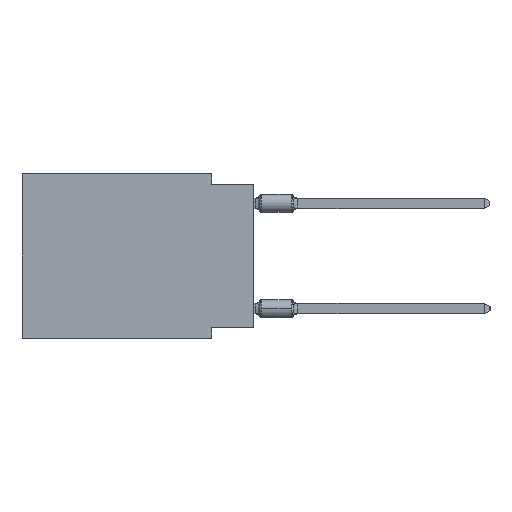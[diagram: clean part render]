
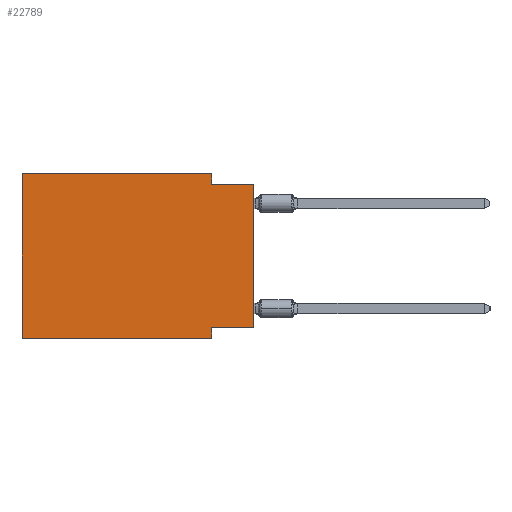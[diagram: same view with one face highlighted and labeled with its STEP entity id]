
A CAD part, left-side view. The second image highlights one B-rep face of the part: STEP entity #22789.
In plain terms, the highlighted planar face has unit normal (-1, 0, 0).
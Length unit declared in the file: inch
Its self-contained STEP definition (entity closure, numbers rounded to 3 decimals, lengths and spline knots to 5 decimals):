
#131 = CARTESIAN_POINT ( 'NONE',  ( 0., 0.1, -0.39 ) ) ;
#593 = LINE ( 'NONE', #9937, #12192 ) ;
#1393 = CARTESIAN_POINT ( 'NONE',  ( 0., 0.1, 0. ) ) ;
#1691 = ORIENTED_EDGE ( 'NONE', *, *, #12600, .F. ) ;
#2046 = ORIENTED_EDGE ( 'NONE', *, *, #15330, .F. ) ;
#2110 = DIRECTION ( 'NONE',  ( 0., 0., -1. ) ) ;
#2387 = VERTEX_POINT ( 'NONE', #2949 ) ;
#2538 = ORIENTED_EDGE ( 'NONE', *, *, #18547, .F. ) ;
#2949 = CARTESIAN_POINT ( 'NONE',  ( 0., 0.55, -0.39 ) ) ;
#3519 = VERTEX_POINT ( 'NONE', #9788 ) ;
#3771 = ORIENTED_EDGE ( 'NONE', *, *, #26966, .F. ) ;
#4099 = LINE ( 'NONE', #29388, #11562 ) ;
#5798 = ORIENTED_EDGE ( 'NONE', *, *, #21967, .T. ) ;
#5980 = ORIENTED_EDGE ( 'NONE', *, *, #15368, .T. ) ;
#7129 = VERTEX_POINT ( 'NONE', #11928 ) ;
#7534 = CARTESIAN_POINT ( 'NONE',  ( 0., 0., -0.365 ) ) ;
#7773 = VECTOR ( 'NONE', #2110, 39.37008 ) ;
#7904 = DIRECTION ( 'NONE',  ( 0., -1., 0. ) ) ;
#8086 = VERTEX_POINT ( 'NONE', #22622 ) ;
#9294 = CARTESIAN_POINT ( 'NONE',  ( 0., 0.1, 0. ) ) ;
#9782 = CARTESIAN_POINT ( 'NONE',  ( 0., 0.55, -0.39 ) ) ;
#9788 = CARTESIAN_POINT ( 'NONE',  ( 0., 0.55, 0. ) ) ;
#9811 = DIRECTION ( 'NONE',  ( 0., 0., 1. ) ) ;
#9903 = EDGE_CURVE ( 'NONE', #2387, #3519, #4099, .T. ) ;
#9937 = CARTESIAN_POINT ( 'NONE',  ( 0., 0., -0.365 ) ) ;
#10056 = VERTEX_POINT ( 'NONE', #27062 ) ;
#10591 = DIRECTION ( 'NONE',  ( 0., 0., -1. ) ) ;
#11188 = DIRECTION ( 'NONE',  ( 0., 0., 1. ) ) ;
#11562 = VECTOR ( 'NONE', #11188, 39.37008 ) ;
#11720 = DIRECTION ( 'NONE',  ( 0., -1., 0. ) ) ;
#11928 = CARTESIAN_POINT ( 'NONE',  ( 0., 0.1, -0.025 ) ) ;
#12192 = VECTOR ( 'NONE', #28292, 39.37008 ) ;
#12600 = EDGE_CURVE ( 'NONE', #20473, #13863, #593, .T. ) ;
#13360 = EDGE_LOOP ( 'NONE', ( #5798, #2538, #3771, #13796, #21833, #5980, #2046, #1691 ) ) ;
#13619 = DIRECTION ( 'NONE',  ( 1., 0., 0. ) ) ;
#13796 = ORIENTED_EDGE ( 'NONE', *, *, #23709, .F. ) ;
#13863 = VERTEX_POINT ( 'NONE', #27448 ) ;
#14271 = VECTOR ( 'NONE', #11720, 39.37008 ) ;
#14648 = LINE ( 'NONE', #16907, #27155 ) ;
#15330 = EDGE_CURVE ( 'NONE', #13863, #10056, #22752, .T. ) ;
#15368 = EDGE_CURVE ( 'NONE', #2387, #10056, #23639, .T. ) ;
#15563 = FACE_OUTER_BOUND ( 'NONE', #13360, .T. ) ;
#16907 = CARTESIAN_POINT ( 'NONE',  ( 0., 0., 0. ) ) ;
#18547 = EDGE_CURVE ( 'NONE', #7129, #8086, #28783, .T. ) ;
#18630 = LINE ( 'NONE', #22714, #14271 ) ;
#19469 = CARTESIAN_POINT ( 'NONE',  ( 0., 0., -0.025 ) ) ;
#19980 = AXIS2_PLACEMENT_3D ( 'NONE', #24577, #13619, #20506 ) ;
#20473 = VERTEX_POINT ( 'NONE', #7534 ) ;
#20506 = DIRECTION ( 'NONE',  ( 0., 0., -1. ) ) ;
#20609 = VECTOR ( 'NONE', #10591, 39.37008 ) ;
#21382 = DIRECTION ( 'NONE',  ( 0., -1., 0. ) ) ;
#21747 = LINE ( 'NONE', #1393, #20609 ) ;
#21833 = ORIENTED_EDGE ( 'NONE', *, *, #9903, .F. ) ;
#21967 = EDGE_CURVE ( 'NONE', #20473, #8086, #14648, .T. ) ;
#22202 = PLANE ( 'NONE',  #19980 ) ;
#22622 = CARTESIAN_POINT ( 'NONE',  ( 0., 0., -0.025 ) ) ;
#22714 = CARTESIAN_POINT ( 'NONE',  ( 0., 0.55, 0. ) ) ;
#22752 = LINE ( 'NONE', #131, #7773 ) ;
#22789 = ADVANCED_FACE ( 'NONE', ( #15563 ), #22202, .F. ) ;
#23639 = LINE ( 'NONE', #9782, #27449 ) ;
#23709 = EDGE_CURVE ( 'NONE', #3519, #23807, #18630, .T. ) ;
#23807 = VERTEX_POINT ( 'NONE', #9294 ) ;
#24577 = CARTESIAN_POINT ( 'NONE',  ( 0., 0.55, 0. ) ) ;
#26966 = EDGE_CURVE ( 'NONE', #23807, #7129, #21747, .T. ) ;
#27062 = CARTESIAN_POINT ( 'NONE',  ( 0., 0.1, -0.39 ) ) ;
#27155 = VECTOR ( 'NONE', #9811, 39.37008 ) ;
#27448 = CARTESIAN_POINT ( 'NONE',  ( 0., 0.1, -0.365 ) ) ;
#27449 = VECTOR ( 'NONE', #21382, 39.37008 ) ;
#28292 = DIRECTION ( 'NONE',  ( 0., 1., 0. ) ) ;
#28783 = LINE ( 'NONE', #19469, #28951 ) ;
#28951 = VECTOR ( 'NONE', #7904, 39.37008 ) ;
#29388 = CARTESIAN_POINT ( 'NONE',  ( 0., 0.55, 0. ) ) ;
